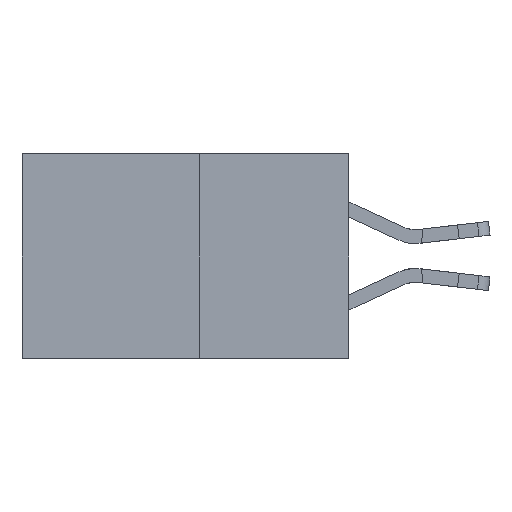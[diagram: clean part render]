
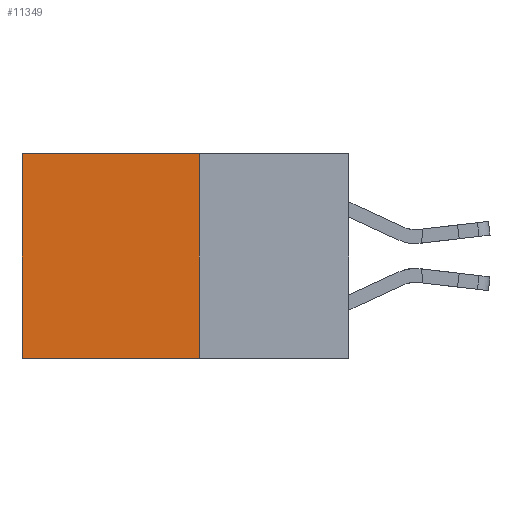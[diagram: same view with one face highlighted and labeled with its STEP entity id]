
A CAD part, left-side view. The second image highlights one B-rep face of the part: STEP entity #11349.
In plain terms, the highlighted planar face has unit normal (-1, 0, 0).
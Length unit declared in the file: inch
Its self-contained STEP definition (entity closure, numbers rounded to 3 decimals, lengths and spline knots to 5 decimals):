
#303 = DIRECTION ( 'NONE',  ( 0., 0., -1. ) ) ;
#915 = LINE ( 'NONE', #9861, #20892 ) ;
#1347 = EDGE_CURVE ( 'NONE', #14374, #3218, #9458, .T. ) ;
#1852 = CARTESIAN_POINT ( 'NONE',  ( 0.277, 0.27, -0.37 ) ) ;
#3218 = VERTEX_POINT ( 'NONE', #21549 ) ;
#3324 = CARTESIAN_POINT ( 'NONE',  ( 0.277, 0.27, -0.37 ) ) ;
#3738 = DIRECTION ( 'NONE',  ( 1., 0., 0. ) ) ;
#3790 = ORIENTED_EDGE ( 'NONE', *, *, #23199, .T. ) ;
#3911 = CARTESIAN_POINT ( 'NONE',  ( 0.277, 0.59, -0.37 ) ) ;
#5007 = CARTESIAN_POINT ( 'NONE',  ( 0.277, 0.27, 0. ) ) ;
#6002 = DIRECTION ( 'NONE',  ( 0., 0., -1. ) ) ;
#6774 = VERTEX_POINT ( 'NONE', #3324 ) ;
#7015 = VECTOR ( 'NONE', #13287, 39.37008 ) ;
#7777 = AXIS2_PLACEMENT_3D ( 'NONE', #1852, #3738, #16857 ) ;
#8577 = EDGE_CURVE ( 'NONE', #6774, #3218, #14192, .T. ) ;
#9458 = LINE ( 'NONE', #3911, #18669 ) ;
#9832 = DIRECTION ( 'NONE',  ( 0., 1., 0. ) ) ;
#9861 = CARTESIAN_POINT ( 'NONE',  ( 0.277, 0.27, -0.37 ) ) ;
#9940 = ORIENTED_EDGE ( 'NONE', *, *, #8577, .F. ) ;
#9989 = CARTESIAN_POINT ( 'NONE',  ( 0.277, 0.27, -0.37 ) ) ;
#11349 = ADVANCED_FACE ( 'NONE', ( #15392 ), #13176, .F. ) ;
#11455 = ORIENTED_EDGE ( 'NONE', *, *, #16844, .F. ) ;
#11470 = ORIENTED_EDGE ( 'NONE', *, *, #1347, .T. ) ;
#13126 = VERTEX_POINT ( 'NONE', #5007 ) ;
#13176 = PLANE ( 'NONE',  #7777 ) ;
#13287 = DIRECTION ( 'NONE',  ( 0., 1., 0. ) ) ;
#13612 = VECTOR ( 'NONE', #9832, 39.37008 ) ;
#14192 = LINE ( 'NONE', #9989, #13612 ) ;
#14374 = VERTEX_POINT ( 'NONE', #17666 ) ;
#15392 = FACE_OUTER_BOUND ( 'NONE', #20564, .T. ) ;
#16844 = EDGE_CURVE ( 'NONE', #13126, #6774, #915, .T. ) ;
#16857 = DIRECTION ( 'NONE',  ( 0., 0., -1. ) ) ;
#16954 = CARTESIAN_POINT ( 'NONE',  ( 0.277, 0.27, 0. ) ) ;
#17666 = CARTESIAN_POINT ( 'NONE',  ( 0.277, 0.59, 0. ) ) ;
#18669 = VECTOR ( 'NONE', #6002, 39.37008 ) ;
#20564 = EDGE_LOOP ( 'NONE', ( #11470, #9940, #11455, #3790 ) ) ;
#20892 = VECTOR ( 'NONE', #303, 39.37008 ) ;
#21549 = CARTESIAN_POINT ( 'NONE',  ( 0.277, 0.59, -0.37 ) ) ;
#22452 = LINE ( 'NONE', #16954, #7015 ) ;
#23199 = EDGE_CURVE ( 'NONE', #13126, #14374, #22452, .T. ) ;
